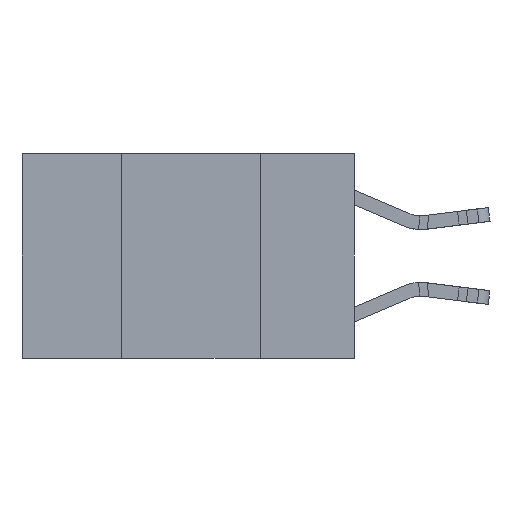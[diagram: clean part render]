
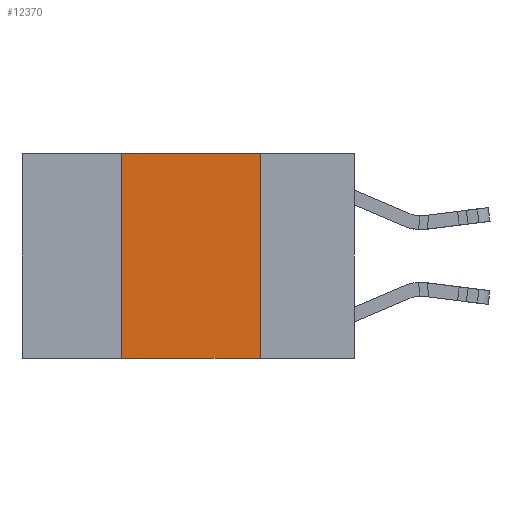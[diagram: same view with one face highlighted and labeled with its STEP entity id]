
A CAD part, left-side view. The second image highlights one B-rep face of the part: STEP entity #12370.
In plain terms, the highlighted planar face has unit normal (-1, 0, 0).
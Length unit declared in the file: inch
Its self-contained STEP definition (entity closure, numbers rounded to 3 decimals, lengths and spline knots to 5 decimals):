
#1029 = VECTOR ( 'NONE', #3920, 39.37008 ) ;
#1394 = VERTEX_POINT ( 'NONE', #14263 ) ;
#1863 = VECTOR ( 'NONE', #21026, 39.37008 ) ;
#2132 = AXIS2_PLACEMENT_3D ( 'NONE', #32166, #17365, #2387 ) ;
#2387 = DIRECTION ( 'NONE',  ( 0., 0., -1. ) ) ;
#2771 = ORIENTED_EDGE ( 'NONE', *, *, #8016, .F. ) ;
#3565 = ORIENTED_EDGE ( 'NONE', *, *, #32116, .F. ) ;
#3916 = CARTESIAN_POINT ( 'NONE',  ( 0., 0.6, 0. ) ) ;
#3920 = DIRECTION ( 'NONE',  ( 0., -1., 0. ) ) ;
#4338 = ORIENTED_EDGE ( 'NONE', *, *, #30225, .T. ) ;
#6014 = VERTEX_POINT ( 'NONE', #9488 ) ;
#8016 = EDGE_CURVE ( 'NONE', #1394, #27358, #28344, .T. ) ;
#9488 = CARTESIAN_POINT ( 'NONE',  ( 0., 0.42, -0.37 ) ) ;
#10438 = CARTESIAN_POINT ( 'NONE',  ( 0., 0.42, 0. ) ) ;
#12370 = ADVANCED_FACE ( 'NONE', ( #20708 ), #19730, .F. ) ;
#12947 = DIRECTION ( 'NONE',  ( 0., 0., 1. ) ) ;
#13188 = EDGE_LOOP ( 'NONE', ( #2771, #16082, #3565, #4338 ) ) ;
#14263 = CARTESIAN_POINT ( 'NONE',  ( 0., 0.17, 0. ) ) ;
#14321 = LINE ( 'NONE', #21347, #1029 ) ;
#14926 = EDGE_CURVE ( 'NONE', #27313, #1394, #27955, .T. ) ;
#16082 = ORIENTED_EDGE ( 'NONE', *, *, #14926, .F. ) ;
#17365 = DIRECTION ( 'NONE',  ( 1., 0., 0. ) ) ;
#17704 = VECTOR ( 'NONE', #12947, 39.37008 ) ;
#19730 = PLANE ( 'NONE',  #2132 ) ;
#20708 = FACE_OUTER_BOUND ( 'NONE', #13188, .T. ) ;
#21026 = DIRECTION ( 'NONE',  ( 0., 0., -1. ) ) ;
#21347 = CARTESIAN_POINT ( 'NONE',  ( 0., 0.6, -0.37 ) ) ;
#22150 = CARTESIAN_POINT ( 'NONE',  ( 0., 0.17, -0.37 ) ) ;
#25895 = CARTESIAN_POINT ( 'NONE',  ( 0., 0.17, 0. ) ) ;
#26904 = CARTESIAN_POINT ( 'NONE',  ( 0., 0.42, 0. ) ) ;
#27313 = VERTEX_POINT ( 'NONE', #26904 ) ;
#27358 = VERTEX_POINT ( 'NONE', #22150 ) ;
#27955 = LINE ( 'NONE', #3916, #28748 ) ;
#28344 = LINE ( 'NONE', #25895, #1863 ) ;
#28748 = VECTOR ( 'NONE', #28830, 39.37008 ) ;
#28830 = DIRECTION ( 'NONE',  ( 0., -1., 0. ) ) ;
#30225 = EDGE_CURVE ( 'NONE', #6014, #27358, #14321, .T. ) ;
#31649 = LINE ( 'NONE', #10438, #17704 ) ;
#32116 = EDGE_CURVE ( 'NONE', #6014, #27313, #31649, .T. ) ;
#32166 = CARTESIAN_POINT ( 'NONE',  ( 0., 0.6, 0. ) ) ;
